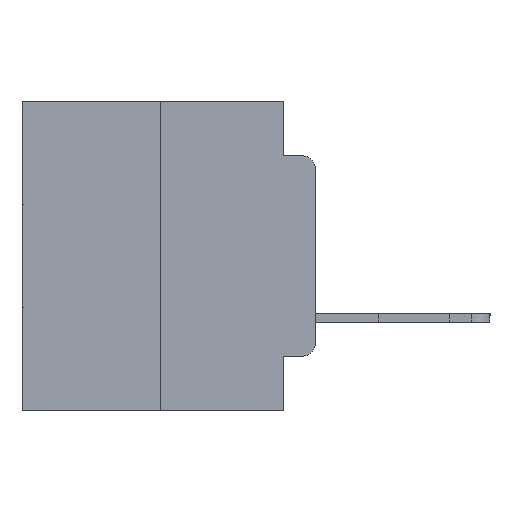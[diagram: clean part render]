
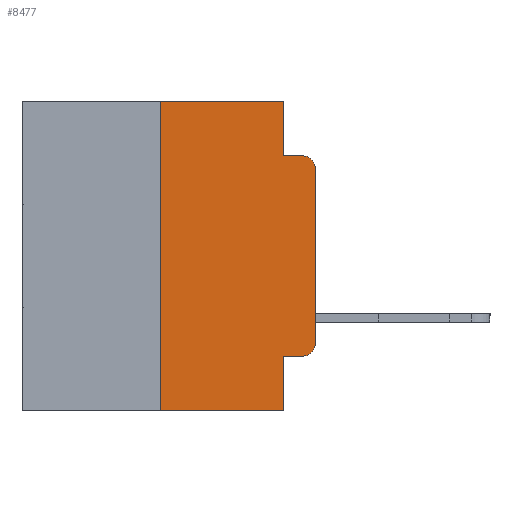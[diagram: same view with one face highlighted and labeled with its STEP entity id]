
A CAD part, left-side view. The second image highlights one B-rep face of the part: STEP entity #8477.
In plain terms, the highlighted planar face has unit normal (-1, 0, 0).
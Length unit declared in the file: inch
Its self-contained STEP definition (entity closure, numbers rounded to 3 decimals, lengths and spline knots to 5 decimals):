
#17 = ORIENTED_EDGE ( 'NONE', *, *, #21075, .F. ) ;
#812 = VERTEX_POINT ( 'NONE', #12250 ) ;
#1068 = VERTEX_POINT ( 'NONE', #11366 ) ;
#1834 = CARTESIAN_POINT ( 'NONE',  ( 0., 0.051, -0.4115 ) ) ;
#2444 = LINE ( 'NONE', #11297, #8715 ) ;
#2618 = DIRECTION ( 'NONE',  ( -1., 0., 0. ) ) ;
#2777 = CARTESIAN_POINT ( 'NONE',  ( 0., 0., -0.1085 ) ) ;
#2898 = CARTESIAN_POINT ( 'NONE',  ( 0., 0.473, -0.5 ) ) ;
#3079 = ORIENTED_EDGE ( 'NONE', *, *, #26278, .F. ) ;
#3315 = CARTESIAN_POINT ( 'NONE',  ( 0., 0.051, 0. ) ) ;
#3334 = VECTOR ( 'NONE', #21593, 39.37008 ) ;
#3700 = VERTEX_POINT ( 'NONE', #18803 ) ;
#3723 = CARTESIAN_POINT ( 'NONE',  ( 0., 0.051, 0. ) ) ;
#4331 = FACE_OUTER_BOUND ( 'NONE', #6583, .T. ) ;
#4362 = CARTESIAN_POINT ( 'NONE',  ( 0., 0.25, 0. ) ) ;
#4934 = VECTOR ( 'NONE', #11886, 39.37008 ) ;
#5069 = VERTEX_POINT ( 'NONE', #2777 ) ;
#5140 = CARTESIAN_POINT ( 'NONE',  ( 0., 0.473, 0. ) ) ;
#6193 = VERTEX_POINT ( 'NONE', #19768 ) ;
#6348 = LINE ( 'NONE', #3723, #3334 ) ;
#6418 = VECTOR ( 'NONE', #17916, 39.37008 ) ;
#6583 = EDGE_LOOP ( 'NONE', ( #21964, #11820, #17652, #17, #13211, #3079, #9370, #20995, #16665, #22303 ) ) ;
#7296 = CARTESIAN_POINT ( 'NONE',  ( 0., 0., -0.3915 ) ) ;
#7310 = CARTESIAN_POINT ( 'NONE',  ( 0., 0.051, -0.4115 ) ) ;
#8352 = VERTEX_POINT ( 'NONE', #28791 ) ;
#8477 = ADVANCED_FACE ( 'NONE', ( #4331 ), #12110, .F. ) ;
#8715 = VECTOR ( 'NONE', #28368, 39.37008 ) ;
#9026 = CARTESIAN_POINT ( 'NONE',  ( 0., 0.051, -0.0885 ) ) ;
#9370 = ORIENTED_EDGE ( 'NONE', *, *, #20455, .T. ) ;
#11007 = EDGE_CURVE ( 'NONE', #21127, #8352, #6348, .T. ) ;
#11127 = LINE ( 'NONE', #7310, #4934 ) ;
#11297 = CARTESIAN_POINT ( 'NONE',  ( 0., 0., 0. ) ) ;
#11366 = CARTESIAN_POINT ( 'NONE',  ( 0., 0.02, -0.4115 ) ) ;
#11433 = VECTOR ( 'NONE', #27136, 39.37008 ) ;
#11820 = ORIENTED_EDGE ( 'NONE', *, *, #25792, .T. ) ;
#11886 = DIRECTION ( 'NONE',  ( 0., -1., 0. ) ) ;
#12097 = VECTOR ( 'NONE', #24268, 39.37008 ) ;
#12110 = PLANE ( 'NONE',  #12937 ) ;
#12203 = AXIS2_PLACEMENT_3D ( 'NONE', #13416, #28375, #15642 ) ;
#12250 = CARTESIAN_POINT ( 'NONE',  ( 0., 0.25, -0.5 ) ) ;
#12289 = LINE ( 'NONE', #21795, #28046 ) ;
#12817 = LINE ( 'NONE', #2898, #11433 ) ;
#12937 = AXIS2_PLACEMENT_3D ( 'NONE', #5140, #27092, #14323 ) ;
#13211 = ORIENTED_EDGE ( 'NONE', *, *, #13895, .F. ) ;
#13416 = CARTESIAN_POINT ( 'NONE',  ( 0., 0.02, -0.3915 ) ) ;
#13895 = EDGE_CURVE ( 'NONE', #24279, #22157, #12289, .T. ) ;
#14323 = DIRECTION ( 'NONE',  ( 0., 0., -1. ) ) ;
#15642 = DIRECTION ( 'NONE',  ( 0., 0., -1. ) ) ;
#16309 = CARTESIAN_POINT ( 'NONE',  ( 0., 0.02, -0.1085 ) ) ;
#16665 = ORIENTED_EDGE ( 'NONE', *, *, #19799, .T. ) ;
#17530 = DIRECTION ( 'NONE',  ( 0., -1., 0. ) ) ;
#17580 = DIRECTION ( 'NONE',  ( 0., 0., -1. ) ) ;
#17652 = ORIENTED_EDGE ( 'NONE', *, *, #20208, .F. ) ;
#17916 = DIRECTION ( 'NONE',  ( 0., -1., 0. ) ) ;
#18353 = EDGE_CURVE ( 'NONE', #23952, #5069, #2444, .T. ) ;
#18477 = DIRECTION ( 'NONE',  ( 0., 0., -1. ) ) ;
#18803 = CARTESIAN_POINT ( 'NONE',  ( 0., 0.02, -0.0885 ) ) ;
#19305 = CIRCLE ( 'NONE', #24919, 0.02 ) ;
#19768 = CARTESIAN_POINT ( 'NONE',  ( 0., 0.051, -0.0885 ) ) ;
#19799 = EDGE_CURVE ( 'NONE', #21127, #1068, #11127, .T. ) ;
#20171 = EDGE_CURVE ( 'NONE', #1068, #23952, #24573, .T. ) ;
#20208 = EDGE_CURVE ( 'NONE', #6193, #3700, #23921, .T. ) ;
#20455 = EDGE_CURVE ( 'NONE', #812, #8352, #12817, .T. ) ;
#20995 = ORIENTED_EDGE ( 'NONE', *, *, #11007, .F. ) ;
#21075 = EDGE_CURVE ( 'NONE', #22157, #6193, #28185, .T. ) ;
#21127 = VERTEX_POINT ( 'NONE', #1834 ) ;
#21517 = CARTESIAN_POINT ( 'NONE',  ( 0., 0.25, 0. ) ) ;
#21593 = DIRECTION ( 'NONE',  ( 0., 0., -1. ) ) ;
#21795 = CARTESIAN_POINT ( 'NONE',  ( 0., 0.473, 0. ) ) ;
#21964 = ORIENTED_EDGE ( 'NONE', *, *, #18353, .T. ) ;
#22157 = VERTEX_POINT ( 'NONE', #3315 ) ;
#22303 = ORIENTED_EDGE ( 'NONE', *, *, #20171, .T. ) ;
#22538 = VECTOR ( 'NONE', #17580, 39.37008 ) ;
#23921 = LINE ( 'NONE', #9026, #6418 ) ;
#23952 = VERTEX_POINT ( 'NONE', #7296 ) ;
#24268 = DIRECTION ( 'NONE',  ( 0., 0., 1. ) ) ;
#24279 = VERTEX_POINT ( 'NONE', #21517 ) ;
#24573 = CIRCLE ( 'NONE', #12203, 0.02 ) ;
#24862 = LINE ( 'NONE', #4362, #12097 ) ;
#24919 = AXIS2_PLACEMENT_3D ( 'NONE', #16309, #2618, #18477 ) ;
#25792 = EDGE_CURVE ( 'NONE', #5069, #3700, #19305, .T. ) ;
#26278 = EDGE_CURVE ( 'NONE', #812, #24279, #24862, .T. ) ;
#27092 = DIRECTION ( 'NONE',  ( 1., 0., 0. ) ) ;
#27136 = DIRECTION ( 'NONE',  ( 0., -1., 0. ) ) ;
#28046 = VECTOR ( 'NONE', #17530, 39.37008 ) ;
#28147 = CARTESIAN_POINT ( 'NONE',  ( 0., 0.051, 0. ) ) ;
#28185 = LINE ( 'NONE', #28147, #22538 ) ;
#28368 = DIRECTION ( 'NONE',  ( 0., 0., 1. ) ) ;
#28375 = DIRECTION ( 'NONE',  ( -1., 0., 0. ) ) ;
#28791 = CARTESIAN_POINT ( 'NONE',  ( 0., 0.051, -0.5 ) ) ;
